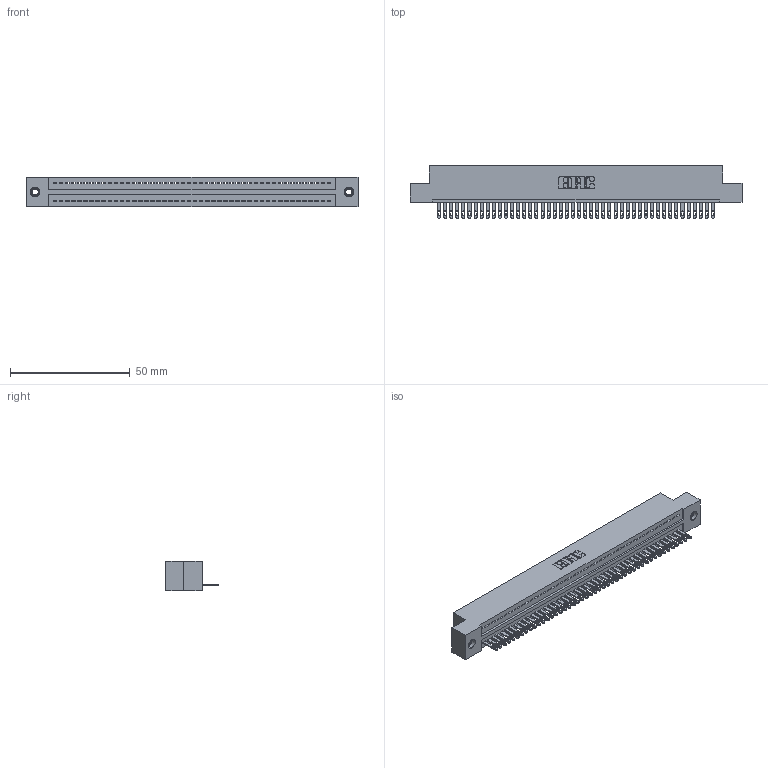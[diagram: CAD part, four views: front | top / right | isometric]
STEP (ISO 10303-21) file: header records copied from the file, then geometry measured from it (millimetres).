
FILE_DESCRIPTION (( 'STEP AP203' ), '1' );
FILE_NAME ('325-046-500-107.STEP', '2020-02-24T22:45:10', ( '' ), ( '' ), 'SwSTEP 2.0', 'SolidWorks 2016', '' );
FILE_SCHEMA (( 'CONFIG_CONTROL_DESIGN' ));
Length unit declared in the file: inch
Products named in the file (4): 345-250-001_345-250-005-103; 325 Part_TI; 325-046-500-107; 325-292-001_325-293-100
Assembly tree (49 placements, depth 2):
  325-046-500-107
    325 Part_TI
    325-292-001_325-293-100  x46
    345-250-001_345-250-005-103  x2
Bounding box: 138.56 x 21.84 x 12.45 mm (x, y, z)
Volume: 17636.3 mm3; surface area: 19470.4 mm2
Topology: 49 solids, 49 shells, 2658 faces, 8175 edges, 5442 vertices
Faces by surface type: plane 1758, cylinder 884, cone 12, torus 4
Entity records: 28720 total; most frequent: CARTESIAN_POINT 4935, ORIENTED_EDGE 4910, DIRECTION 4189, EDGE_CURVE 2455, LINE 2303, VECTOR 2303, VERTEX_POINT 1632, AXIS2_PLACEMENT_3D 943
